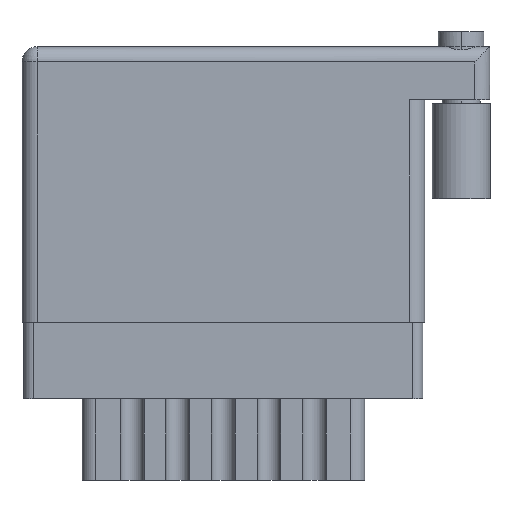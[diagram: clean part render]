
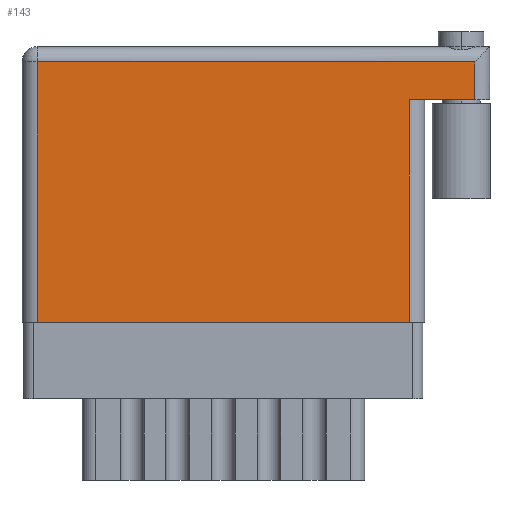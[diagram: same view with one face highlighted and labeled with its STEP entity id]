
A CAD part, front view. The second image highlights one B-rep face of the part: STEP entity #143.
In plain terms, the highlighted face is planar.
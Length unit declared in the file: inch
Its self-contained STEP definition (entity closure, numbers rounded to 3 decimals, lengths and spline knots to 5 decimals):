
#65 = VERTEX_POINT ( 'NONE', #13629 ) ;
#143 = ADVANCED_FACE ( 'NONE', ( #2139 ), #2395, .F. ) ;
#1207 = ORIENTED_EDGE ( 'NONE', *, *, #6096, .T. ) ;
#1437 = CARTESIAN_POINT ( 'NONE',  ( 1.489, 0.906, 0. ) ) ;
#2139 = FACE_OUTER_BOUND ( 'NONE', #5640, .T. ) ;
#2264 = DIRECTION ( 'NONE',  ( -1., 0., 0. ) ) ;
#2395 = PLANE ( 'NONE',  #14511 ) ;
#2919 = EDGE_CURVE ( 'NONE', #17351, #10769, #22909, .T. ) ;
#4540 = EDGE_CURVE ( 'NONE', #5696, #65, #15102, .T. ) ;
#4557 = CARTESIAN_POINT ( 'NONE',  ( 0.05, 0., 0. ) ) ;
#4741 = ORIENTED_EDGE ( 'NONE', *, *, #14450, .F. ) ;
#5640 = EDGE_LOOP ( 'NONE', ( #1207, #23987, #4741, #9646, #6469, #19532 ) ) ;
#5696 = VERTEX_POINT ( 'NONE', #24682 ) ;
#6096 = EDGE_CURVE ( 'NONE', #6284, #5696, #23737, .T. ) ;
#6284 = VERTEX_POINT ( 'NONE', #4557 ) ;
#6399 = DIRECTION ( 'NONE',  ( 0., -1., 0. ) ) ;
#6469 = ORIENTED_EDGE ( 'NONE', *, *, #2919, .T. ) ;
#6750 = DIRECTION ( 'NONE',  ( -1., 0., 0. ) ) ;
#6773 = CARTESIAN_POINT ( 'NONE',  ( 0., 0.856, 0. ) ) ;
#6794 = CARTESIAN_POINT ( 'NONE',  ( 0.05, 0., 0. ) ) ;
#7043 = VECTOR ( 'NONE', #22786, 39.37008 ) ;
#9646 = ORIENTED_EDGE ( 'NONE', *, *, #14994, .T. ) ;
#9999 = CARTESIAN_POINT ( 'NONE',  ( 1.489, 0.856, 0. ) ) ;
#10281 = CARTESIAN_POINT ( 'NONE',  ( 1.489, 0.731, 0. ) ) ;
#10769 = VERTEX_POINT ( 'NONE', #23015 ) ;
#10932 = DIRECTION ( 'NONE',  ( 0., 1., 0. ) ) ;
#11056 = LINE ( 'NONE', #1437, #25025 ) ;
#11683 = DIRECTION ( 'NONE',  ( 1., 0., 0. ) ) ;
#12395 = CARTESIAN_POINT ( 'NONE',  ( 0., 0.906, 0. ) ) ;
#13250 = DIRECTION ( 'NONE',  ( 0., 1., 0. ) ) ;
#13629 = CARTESIAN_POINT ( 'NONE',  ( 1.275, 0.731, 0. ) ) ;
#13955 = VECTOR ( 'NONE', #6750, 39.37008 ) ;
#14388 = CARTESIAN_POINT ( 'NONE',  ( 1.539, 0.731, 0. ) ) ;
#14450 = EDGE_CURVE ( 'NONE', #14760, #65, #24742, .T. ) ;
#14511 = AXIS2_PLACEMENT_3D ( 'NONE', #12395, #16217, #2264 ) ;
#14760 = VERTEX_POINT ( 'NONE', #10281 ) ;
#14994 = EDGE_CURVE ( 'NONE', #14760, #17351, #11056, .T. ) ;
#15102 = LINE ( 'NONE', #19032, #16069 ) ;
#16069 = VECTOR ( 'NONE', #13250, 39.37008 ) ;
#16217 = DIRECTION ( 'NONE',  ( 0., 0., -1. ) ) ;
#17351 = VERTEX_POINT ( 'NONE', #9999 ) ;
#17841 = CARTESIAN_POINT ( 'NONE',  ( 0., 0., 0. ) ) ;
#18614 = VECTOR ( 'NONE', #11683, 39.37008 ) ;
#19032 = CARTESIAN_POINT ( 'NONE',  ( 1.275, 0.731, 0. ) ) ;
#19532 = ORIENTED_EDGE ( 'NONE', *, *, #19930, .T. ) ;
#19710 = VECTOR ( 'NONE', #6399, 39.37008 ) ;
#19930 = EDGE_CURVE ( 'NONE', #10769, #6284, #22411, .T. ) ;
#22411 = LINE ( 'NONE', #6794, #19710 ) ;
#22786 = DIRECTION ( 'NONE',  ( -1., 0., 0. ) ) ;
#22909 = LINE ( 'NONE', #6773, #7043 ) ;
#23015 = CARTESIAN_POINT ( 'NONE',  ( 0.05, 0.856, 0. ) ) ;
#23737 = LINE ( 'NONE', #17841, #18614 ) ;
#23987 = ORIENTED_EDGE ( 'NONE', *, *, #4540, .T. ) ;
#24682 = CARTESIAN_POINT ( 'NONE',  ( 1.275, 0., 0. ) ) ;
#24742 = LINE ( 'NONE', #14388, #13955 ) ;
#25025 = VECTOR ( 'NONE', #10932, 39.37008 ) ;
